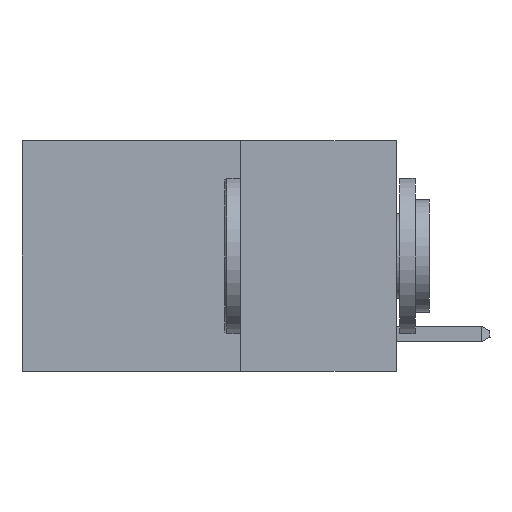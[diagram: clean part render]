
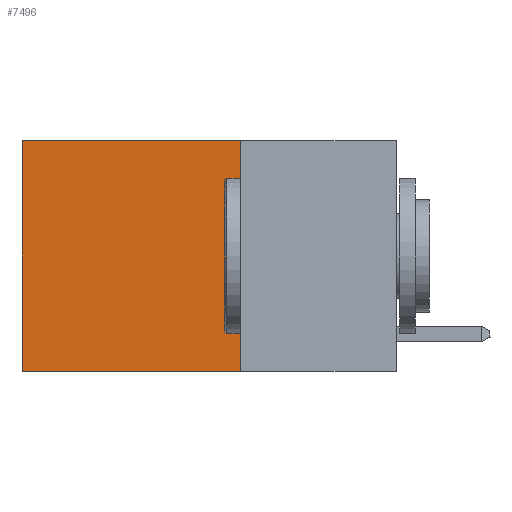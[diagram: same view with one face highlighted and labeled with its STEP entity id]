
A CAD part, left-side view. The second image highlights one B-rep face of the part: STEP entity #7496.
In plain terms, the highlighted planar face has unit normal (-1, 0, 0).
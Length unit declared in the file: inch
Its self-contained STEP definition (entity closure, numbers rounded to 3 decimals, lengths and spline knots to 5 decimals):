
#20 = LINE ( 'NONE', #6075, #8884 ) ;
#1394 = FACE_OUTER_BOUND ( 'NONE', #9650, .T. ) ;
#1811 = DIRECTION ( 'NONE',  ( 0., 1., 0. ) ) ;
#1915 = ORIENTED_EDGE ( 'NONE', *, *, #3795, .T. ) ;
#2206 = PLANE ( 'NONE',  #6085 ) ;
#2751 = EDGE_CURVE ( 'NONE', #13346, #6558, #12038, .T. ) ;
#2782 = VECTOR ( 'NONE', #2838, 39.37008 ) ;
#2797 = ORIENTED_EDGE ( 'NONE', *, *, #2751, .T. ) ;
#2838 = DIRECTION ( 'NONE',  ( 0., 0., -1. ) ) ;
#3219 = CARTESIAN_POINT ( 'NONE',  ( 0.2625, 0.25, -0.37 ) ) ;
#3276 = ORIENTED_EDGE ( 'NONE', *, *, #4539, .F. ) ;
#3744 = EDGE_CURVE ( 'NONE', #11538, #7785, #11504, .T. ) ;
#3795 = EDGE_CURVE ( 'NONE', #11538, #13346, #20, .T. ) ;
#3805 = CARTESIAN_POINT ( 'NONE',  ( 0.2625, 0.6, 0. ) ) ;
#4035 = CARTESIAN_POINT ( 'NONE',  ( 0.2625, 0.25, 0. ) ) ;
#4539 = EDGE_CURVE ( 'NONE', #7785, #6558, #6782, .T. ) ;
#4903 = CARTESIAN_POINT ( 'NONE',  ( 0.2625, 0.6, 0. ) ) ;
#5560 = CARTESIAN_POINT ( 'NONE',  ( 0.2625, 0.25, 0. ) ) ;
#5882 = ORIENTED_EDGE ( 'NONE', *, *, #3744, .F. ) ;
#6075 = CARTESIAN_POINT ( 'NONE',  ( 0.2625, 0.25, 0. ) ) ;
#6085 = AXIS2_PLACEMENT_3D ( 'NONE', #5560, #10570, #9750 ) ;
#6558 = VERTEX_POINT ( 'NONE', #10681 ) ;
#6782 = LINE ( 'NONE', #13068, #11086 ) ;
#6831 = VECTOR ( 'NONE', #10210, 39.37008 ) ;
#7496 = ADVANCED_FACE ( 'NONE', ( #1394 ), #2206, .F. ) ;
#7785 = VERTEX_POINT ( 'NONE', #3219 ) ;
#8884 = VECTOR ( 'NONE', #11357, 39.37008 ) ;
#9650 = EDGE_LOOP ( 'NONE', ( #2797, #3276, #5882, #1915 ) ) ;
#9750 = DIRECTION ( 'NONE',  ( 0., 0., -1. ) ) ;
#10210 = DIRECTION ( 'NONE',  ( 0., 0., -1. ) ) ;
#10570 = DIRECTION ( 'NONE',  ( 1., 0., 0. ) ) ;
#10681 = CARTESIAN_POINT ( 'NONE',  ( 0.2625, 0.6, -0.37 ) ) ;
#10853 = CARTESIAN_POINT ( 'NONE',  ( 0.2625, 0.25, 0. ) ) ;
#11086 = VECTOR ( 'NONE', #1811, 39.37008 ) ;
#11357 = DIRECTION ( 'NONE',  ( 0., 1., 0. ) ) ;
#11504 = LINE ( 'NONE', #4035, #6831 ) ;
#11538 = VERTEX_POINT ( 'NONE', #10853 ) ;
#12038 = LINE ( 'NONE', #3805, #2782 ) ;
#13068 = CARTESIAN_POINT ( 'NONE',  ( 0.2625, 0.25, -0.37 ) ) ;
#13346 = VERTEX_POINT ( 'NONE', #4903 ) ;
